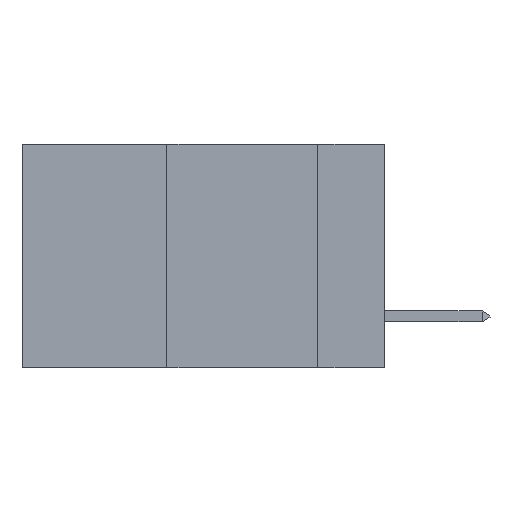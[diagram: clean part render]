
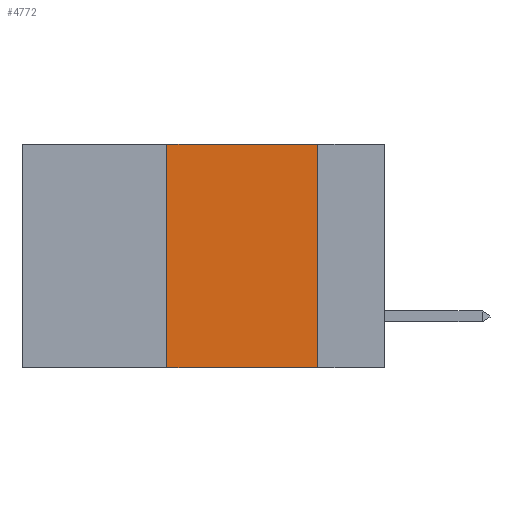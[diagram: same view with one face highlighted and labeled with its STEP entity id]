
A CAD part, left-side view. The second image highlights one B-rep face of the part: STEP entity #4772.
In plain terms, the highlighted planar face has unit normal (-1, 0, 0).
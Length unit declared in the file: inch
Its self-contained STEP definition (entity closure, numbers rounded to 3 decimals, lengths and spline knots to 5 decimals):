
#699 = VERTEX_POINT ( 'NONE', #4571 ) ;
#724 = EDGE_CURVE ( 'NONE', #699, #5621, #2730, .T. ) ;
#818 = VERTEX_POINT ( 'NONE', #3185 ) ;
#842 = VECTOR ( 'NONE', #6991, 39.37008 ) ;
#1446 = DIRECTION ( 'NONE',  ( 1., 0., 0. ) ) ;
#1484 = CARTESIAN_POINT ( 'NONE',  ( 0., 0.6, 0. ) ) ;
#1489 = DIRECTION ( 'NONE',  ( 0., -1., 0. ) ) ;
#1932 = EDGE_CURVE ( 'NONE', #2394, #699, #2290, .T. ) ;
#2290 = LINE ( 'NONE', #1484, #4282 ) ;
#2388 = CARTESIAN_POINT ( 'NONE',  ( 0., 0.6, 0. ) ) ;
#2394 = VERTEX_POINT ( 'NONE', #7128 ) ;
#2553 = ORIENTED_EDGE ( 'NONE', *, *, #724, .F. ) ;
#2730 = LINE ( 'NONE', #10902, #7066 ) ;
#3092 = FACE_OUTER_BOUND ( 'NONE', #5433, .T. ) ;
#3185 = CARTESIAN_POINT ( 'NONE',  ( 0., 0.36, -0.37 ) ) ;
#4282 = VECTOR ( 'NONE', #1489, 39.37008 ) ;
#4323 = CARTESIAN_POINT ( 'NONE',  ( 0., 0.11, -0.37 ) ) ;
#4374 = LINE ( 'NONE', #6632, #8720 ) ;
#4571 = CARTESIAN_POINT ( 'NONE',  ( 0., 0.11, 0. ) ) ;
#4772 = ADVANCED_FACE ( 'NONE', ( #3092 ), #6753, .F. ) ;
#5353 = ORIENTED_EDGE ( 'NONE', *, *, #9822, .F. ) ;
#5433 = EDGE_LOOP ( 'NONE', ( #2553, #9413, #5353, #5633 ) ) ;
#5608 = EDGE_CURVE ( 'NONE', #818, #5621, #7928, .T. ) ;
#5621 = VERTEX_POINT ( 'NONE', #4323 ) ;
#5633 = ORIENTED_EDGE ( 'NONE', *, *, #5608, .T. ) ;
#5809 = DIRECTION ( 'NONE',  ( 0., 0., -1. ) ) ;
#6094 = CARTESIAN_POINT ( 'NONE',  ( 0., 0.6, -0.37 ) ) ;
#6632 = CARTESIAN_POINT ( 'NONE',  ( 0., 0.36, 0. ) ) ;
#6753 = PLANE ( 'NONE',  #9726 ) ;
#6991 = DIRECTION ( 'NONE',  ( 0., -1., 0. ) ) ;
#7066 = VECTOR ( 'NONE', #5809, 39.37008 ) ;
#7128 = CARTESIAN_POINT ( 'NONE',  ( 0., 0.36, 0. ) ) ;
#7483 = DIRECTION ( 'NONE',  ( 0., 0., 1. ) ) ;
#7593 = DIRECTION ( 'NONE',  ( 0., 0., -1. ) ) ;
#7928 = LINE ( 'NONE', #6094, #842 ) ;
#8720 = VECTOR ( 'NONE', #7483, 39.37008 ) ;
#9413 = ORIENTED_EDGE ( 'NONE', *, *, #1932, .F. ) ;
#9726 = AXIS2_PLACEMENT_3D ( 'NONE', #2388, #1446, #7593 ) ;
#9822 = EDGE_CURVE ( 'NONE', #818, #2394, #4374, .T. ) ;
#10902 = CARTESIAN_POINT ( 'NONE',  ( 0., 0.11, 0. ) ) ;
